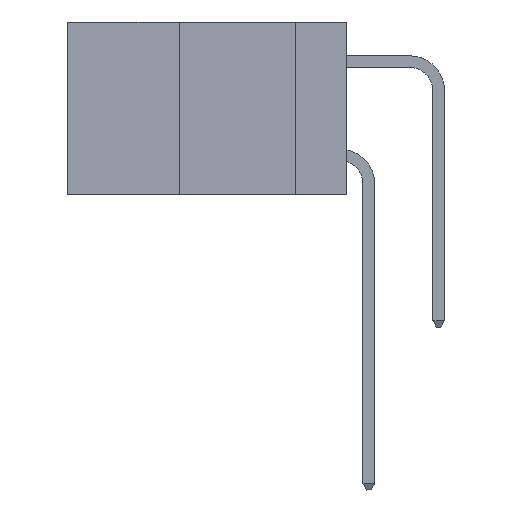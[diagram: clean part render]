
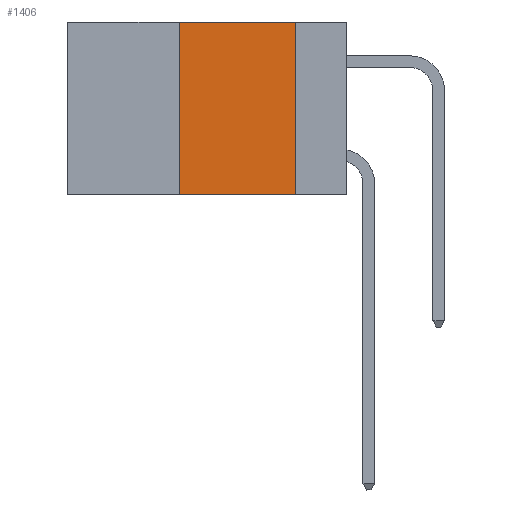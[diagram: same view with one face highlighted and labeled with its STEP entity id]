
A CAD part, left-side view. The second image highlights one B-rep face of the part: STEP entity #1406.
In plain terms, the highlighted planar face has unit normal (-1, 0, 0).
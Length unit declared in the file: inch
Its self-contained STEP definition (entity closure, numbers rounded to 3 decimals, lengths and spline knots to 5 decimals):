
#354 = FACE_OUTER_BOUND ( 'NONE', #8655, .T. ) ;
#809 = VERTEX_POINT ( 'NONE', #3231 ) ;
#979 = DIRECTION ( 'NONE',  ( 0., 0., -1. ) ) ;
#1005 = ORIENTED_EDGE ( 'NONE', *, *, #3758, .F. ) ;
#1406 = ADVANCED_FACE ( 'NONE', ( #354 ), #2199, .F. ) ;
#1559 = LINE ( 'NONE', #12944, #4733 ) ;
#1951 = CARTESIAN_POINT ( 'NONE',  ( 0., 0.6, 0. ) ) ;
#2199 = PLANE ( 'NONE',  #15221 ) ;
#3231 = CARTESIAN_POINT ( 'NONE',  ( 0., 0.36, 0. ) ) ;
#3341 = DIRECTION ( 'NONE',  ( 0., 0., 1. ) ) ;
#3758 = EDGE_CURVE ( 'NONE', #809, #6461, #1559, .T. ) ;
#4733 = VECTOR ( 'NONE', #13209, 39.37008 ) ;
#6461 = VERTEX_POINT ( 'NONE', #35728 ) ;
#8655 = EDGE_LOOP ( 'NONE', ( #24874, #1005, #12341, #36391 ) ) ;
#8844 = CARTESIAN_POINT ( 'NONE',  ( 0., 0.11, -0.37 ) ) ;
#10517 = LINE ( 'NONE', #17546, #36526 ) ;
#12341 = ORIENTED_EDGE ( 'NONE', *, *, #20070, .F. ) ;
#12745 = VERTEX_POINT ( 'NONE', #8844 ) ;
#12944 = CARTESIAN_POINT ( 'NONE',  ( 0., 0.6, 0. ) ) ;
#13209 = DIRECTION ( 'NONE',  ( 0., -1., 0. ) ) ;
#13540 = DIRECTION ( 'NONE',  ( 0., -1., 0. ) ) ;
#13800 = LINE ( 'NONE', #18573, #28575 ) ;
#15221 = AXIS2_PLACEMENT_3D ( 'NONE', #1951, #24820, #22329 ) ;
#17546 = CARTESIAN_POINT ( 'NONE',  ( 0., 0.36, 0. ) ) ;
#18573 = CARTESIAN_POINT ( 'NONE',  ( 0., 0.11, 0. ) ) ;
#20070 = EDGE_CURVE ( 'NONE', #27216, #809, #10517, .T. ) ;
#20609 = VECTOR ( 'NONE', #13540, 39.37008 ) ;
#22329 = DIRECTION ( 'NONE',  ( 0., 0., -1. ) ) ;
#22662 = EDGE_CURVE ( 'NONE', #6461, #12745, #13800, .T. ) ;
#24203 = CARTESIAN_POINT ( 'NONE',  ( 0., 0.36, -0.37 ) ) ;
#24820 = DIRECTION ( 'NONE',  ( 1., 0., 0. ) ) ;
#24874 = ORIENTED_EDGE ( 'NONE', *, *, #22662, .F. ) ;
#25188 = EDGE_CURVE ( 'NONE', #27216, #12745, #35406, .T. ) ;
#27216 = VERTEX_POINT ( 'NONE', #24203 ) ;
#28069 = CARTESIAN_POINT ( 'NONE',  ( 0., 0.6, -0.37 ) ) ;
#28575 = VECTOR ( 'NONE', #979, 39.37008 ) ;
#35406 = LINE ( 'NONE', #28069, #20609 ) ;
#35728 = CARTESIAN_POINT ( 'NONE',  ( 0., 0.11, 0. ) ) ;
#36391 = ORIENTED_EDGE ( 'NONE', *, *, #25188, .T. ) ;
#36526 = VECTOR ( 'NONE', #3341, 39.37008 ) ;
